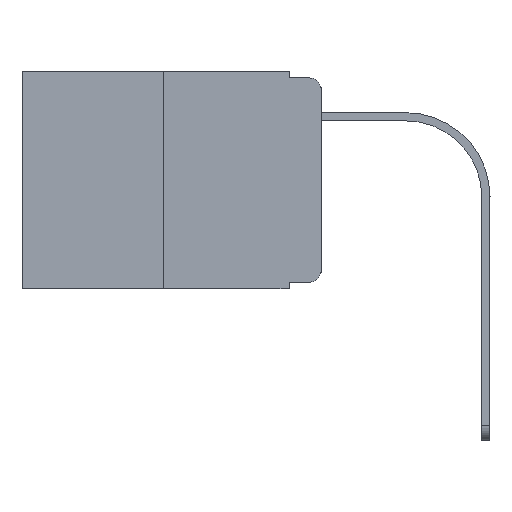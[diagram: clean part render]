
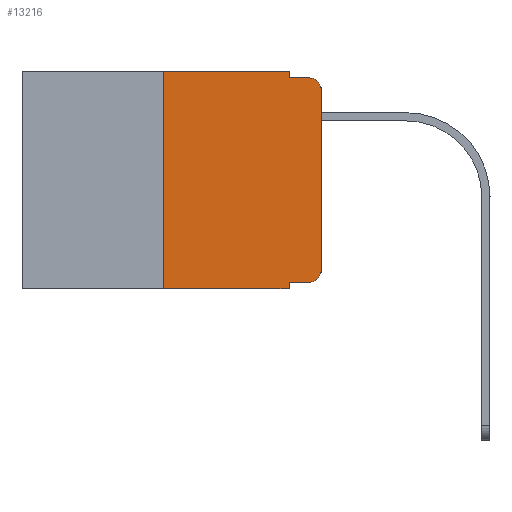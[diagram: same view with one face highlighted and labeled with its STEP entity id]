
A CAD part, left-side view. The second image highlights one B-rep face of the part: STEP entity #13216.
In plain terms, the highlighted planar face has unit normal (-1, 0, 0).
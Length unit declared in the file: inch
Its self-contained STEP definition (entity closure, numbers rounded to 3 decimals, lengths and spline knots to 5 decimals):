
#112 = LINE ( 'NONE', #5361, #11223 ) ;
#159 = ORIENTED_EDGE ( 'NONE', *, *, #7236, .T. ) ;
#424 = CARTESIAN_POINT ( 'NONE',  ( 0., 0.051, 0. ) ) ;
#474 = VECTOR ( 'NONE', #14219, 39.37008 ) ;
#485 = CIRCLE ( 'NONE', #10669, 0.02 ) ;
#620 = DIRECTION ( 'NONE',  ( 0., -1., 0. ) ) ;
#661 = DIRECTION ( 'NONE',  ( 1., 0., 0. ) ) ;
#684 = LINE ( 'NONE', #7040, #13561 ) ;
#813 = CARTESIAN_POINT ( 'NONE',  ( 0., 0.051, 0. ) ) ;
#953 = LINE ( 'NONE', #4825, #15418 ) ;
#1330 = ORIENTED_EDGE ( 'NONE', *, *, #11436, .F. ) ;
#1341 = EDGE_CURVE ( 'NONE', #4625, #15585, #112, .T. ) ;
#1612 = VECTOR ( 'NONE', #11405, 39.37008 ) ;
#1745 = CARTESIAN_POINT ( 'NONE',  ( 0., 0.02, -0.333 ) ) ;
#2053 = ORIENTED_EDGE ( 'NONE', *, *, #8914, .F. ) ;
#2088 = EDGE_CURVE ( 'NONE', #15585, #14882, #15088, .T. ) ;
#2393 = DIRECTION ( 'NONE',  ( -1., 0., 0. ) ) ;
#2496 = ORIENTED_EDGE ( 'NONE', *, *, #2088, .T. ) ;
#2854 = ORIENTED_EDGE ( 'NONE', *, *, #11763, .F. ) ;
#2893 = CARTESIAN_POINT ( 'NONE',  ( 0., 0.051, -0.343 ) ) ;
#3010 = VERTEX_POINT ( 'NONE', #11914 ) ;
#3181 = CARTESIAN_POINT ( 'NONE',  ( 0., 0., 0. ) ) ;
#3650 = DIRECTION ( 'NONE',  ( -1., 0., 0. ) ) ;
#3748 = CARTESIAN_POINT ( 'NONE',  ( 0., 0., -0.313 ) ) ;
#4120 = VECTOR ( 'NONE', #11985, 39.37008 ) ;
#4159 = AXIS2_PLACEMENT_3D ( 'NONE', #7102, #661, #5992 ) ;
#4381 = VERTEX_POINT ( 'NONE', #12977 ) ;
#4616 = PLANE ( 'NONE',  #4159 ) ;
#4625 = VERTEX_POINT ( 'NONE', #12766 ) ;
#4635 = ORIENTED_EDGE ( 'NONE', *, *, #9339, .T. ) ;
#4825 = CARTESIAN_POINT ( 'NONE',  ( 0., 0.051, -0.01 ) ) ;
#4857 = VERTEX_POINT ( 'NONE', #2893 ) ;
#5030 = VERTEX_POINT ( 'NONE', #12741 ) ;
#5361 = CARTESIAN_POINT ( 'NONE',  ( 0., 0.051, -0.333 ) ) ;
#5992 = DIRECTION ( 'NONE',  ( 0., 0., -1. ) ) ;
#6165 = ORIENTED_EDGE ( 'NONE', *, *, #9997, .T. ) ;
#6322 = DIRECTION ( 'NONE',  ( 0., 0., -1. ) ) ;
#6602 = CARTESIAN_POINT ( 'NONE',  ( 0., 0.02, -0.313 ) ) ;
#6737 = VECTOR ( 'NONE', #10000, 39.37008 ) ;
#7040 = CARTESIAN_POINT ( 'NONE',  ( 0., 0.051, 0. ) ) ;
#7102 = CARTESIAN_POINT ( 'NONE',  ( 0., 0.473, 0. ) ) ;
#7236 = EDGE_CURVE ( 'NONE', #3010, #4857, #13897, .T. ) ;
#7307 = CARTESIAN_POINT ( 'NONE',  ( 0., 0.473, -0.343 ) ) ;
#7439 = VECTOR ( 'NONE', #13182, 39.37008 ) ;
#7623 = AXIS2_PLACEMENT_3D ( 'NONE', #6602, #2393, #14410 ) ;
#8028 = VERTEX_POINT ( 'NONE', #813 ) ;
#8914 = EDGE_CURVE ( 'NONE', #3010, #12624, #12827, .T. ) ;
#9179 = CARTESIAN_POINT ( 'NONE',  ( 0., 0.25, 0. ) ) ;
#9185 = EDGE_LOOP ( 'NONE', ( #6165, #4635, #13860, #14911, #2854, #2053, #159, #1330, #11023, #2496 ) ) ;
#9339 = EDGE_CURVE ( 'NONE', #5030, #4381, #485, .T. ) ;
#9356 = VERTEX_POINT ( 'NONE', #10298 ) ;
#9997 = EDGE_CURVE ( 'NONE', #14882, #5030, #11318, .T. ) ;
#10000 = DIRECTION ( 'NONE',  ( 0., -1., 0. ) ) ;
#10004 = EDGE_CURVE ( 'NONE', #9356, #4381, #953, .T. ) ;
#10095 = DIRECTION ( 'NONE',  ( 0., -1., 0. ) ) ;
#10298 = CARTESIAN_POINT ( 'NONE',  ( 0., 0.051, -0.01 ) ) ;
#10669 = AXIS2_PLACEMENT_3D ( 'NONE', #11523, #3650, #6322 ) ;
#11023 = ORIENTED_EDGE ( 'NONE', *, *, #1341, .T. ) ;
#11223 = VECTOR ( 'NONE', #620, 39.37008 ) ;
#11318 = LINE ( 'NONE', #3181, #1612 ) ;
#11405 = DIRECTION ( 'NONE',  ( 0., 0., 1. ) ) ;
#11436 = EDGE_CURVE ( 'NONE', #4625, #4857, #16283, .T. ) ;
#11523 = CARTESIAN_POINT ( 'NONE',  ( 0., 0.02, -0.03 ) ) ;
#11763 = EDGE_CURVE ( 'NONE', #12624, #8028, #16956, .T. ) ;
#11914 = CARTESIAN_POINT ( 'NONE',  ( 0., 0.25, -0.343 ) ) ;
#11985 = DIRECTION ( 'NONE',  ( 0., 0., -1. ) ) ;
#12563 = FACE_OUTER_BOUND ( 'NONE', #9185, .T. ) ;
#12624 = VERTEX_POINT ( 'NONE', #14922 ) ;
#12741 = CARTESIAN_POINT ( 'NONE',  ( 0., 0., -0.03 ) ) ;
#12766 = CARTESIAN_POINT ( 'NONE',  ( 0., 0.051, -0.333 ) ) ;
#12827 = LINE ( 'NONE', #9179, #474 ) ;
#12977 = CARTESIAN_POINT ( 'NONE',  ( 0., 0.02, -0.01 ) ) ;
#13182 = DIRECTION ( 'NONE',  ( 0., -1., 0. ) ) ;
#13216 = ADVANCED_FACE ( 'NONE', ( #12563 ), #4616, .F. ) ;
#13561 = VECTOR ( 'NONE', #14842, 39.37008 ) ;
#13860 = ORIENTED_EDGE ( 'NONE', *, *, #10004, .F. ) ;
#13897 = LINE ( 'NONE', #7307, #6737 ) ;
#14219 = DIRECTION ( 'NONE',  ( 0., 0., 1. ) ) ;
#14280 = EDGE_CURVE ( 'NONE', #8028, #9356, #684, .T. ) ;
#14410 = DIRECTION ( 'NONE',  ( 0., 0., -1. ) ) ;
#14485 = CARTESIAN_POINT ( 'NONE',  ( 0., 0.473, 0. ) ) ;
#14842 = DIRECTION ( 'NONE',  ( 0., 0., -1. ) ) ;
#14882 = VERTEX_POINT ( 'NONE', #3748 ) ;
#14911 = ORIENTED_EDGE ( 'NONE', *, *, #14280, .F. ) ;
#14922 = CARTESIAN_POINT ( 'NONE',  ( 0., 0.25, 0. ) ) ;
#15088 = CIRCLE ( 'NONE', #7623, 0.02 ) ;
#15418 = VECTOR ( 'NONE', #10095, 39.37008 ) ;
#15585 = VERTEX_POINT ( 'NONE', #1745 ) ;
#16283 = LINE ( 'NONE', #424, #4120 ) ;
#16956 = LINE ( 'NONE', #14485, #7439 ) ;
